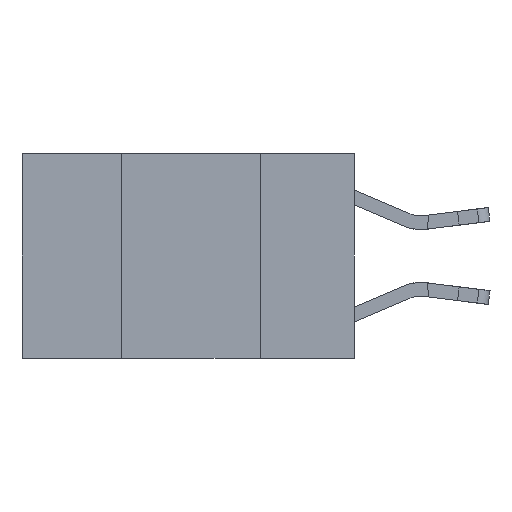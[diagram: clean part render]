
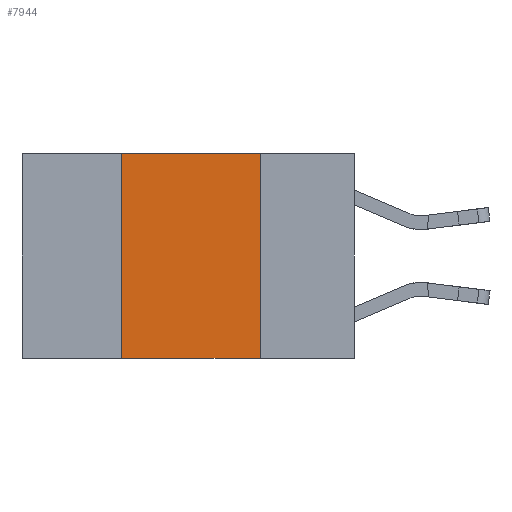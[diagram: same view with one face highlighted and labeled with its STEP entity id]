
A CAD part, left-side view. The second image highlights one B-rep face of the part: STEP entity #7944.
In plain terms, the highlighted planar face has unit normal (-1, 0, 0).
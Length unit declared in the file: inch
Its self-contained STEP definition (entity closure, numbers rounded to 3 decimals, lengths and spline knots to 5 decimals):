
#460 = AXIS2_PLACEMENT_3D ( 'NONE', #2028, #8259, #6343 ) ;
#480 = EDGE_LOOP ( 'NONE', ( #15426, #9861, #7995, #4561 ) ) ;
#1765 = CARTESIAN_POINT ( 'NONE',  ( 0., 0.42, -0.37 ) ) ;
#1944 = EDGE_CURVE ( 'NONE', #5459, #6682, #3910, .T. ) ;
#2028 = CARTESIAN_POINT ( 'NONE',  ( 0., 0.6, 0. ) ) ;
#2651 = CARTESIAN_POINT ( 'NONE',  ( 0., 0.42, 0. ) ) ;
#2825 = LINE ( 'NONE', #9179, #18843 ) ;
#3751 = DIRECTION ( 'NONE',  ( 0., 0., 1. ) ) ;
#3910 = LINE ( 'NONE', #19514, #7775 ) ;
#4037 = LINE ( 'NONE', #16080, #9561 ) ;
#4561 = ORIENTED_EDGE ( 'NONE', *, *, #10125, .T. ) ;
#5097 = FACE_OUTER_BOUND ( 'NONE', #480, .T. ) ;
#5459 = VERTEX_POINT ( 'NONE', #14041 ) ;
#6343 = DIRECTION ( 'NONE',  ( 0., 0., -1. ) ) ;
#6682 = VERTEX_POINT ( 'NONE', #13306 ) ;
#7086 = DIRECTION ( 'NONE',  ( 0., 0., -1. ) ) ;
#7775 = VECTOR ( 'NONE', #7086, 39.37008 ) ;
#7944 = ADVANCED_FACE ( 'NONE', ( #5097 ), #15928, .F. ) ;
#7995 = ORIENTED_EDGE ( 'NONE', *, *, #13094, .F. ) ;
#8259 = DIRECTION ( 'NONE',  ( 1., 0., 0. ) ) ;
#9179 = CARTESIAN_POINT ( 'NONE',  ( 0., 0.6, -0.37 ) ) ;
#9561 = VECTOR ( 'NONE', #19205, 39.37008 ) ;
#9861 = ORIENTED_EDGE ( 'NONE', *, *, #10482, .F. ) ;
#10125 = EDGE_CURVE ( 'NONE', #13511, #6682, #2825, .T. ) ;
#10482 = EDGE_CURVE ( 'NONE', #17206, #5459, #4037, .T. ) ;
#10518 = DIRECTION ( 'NONE',  ( 0., -1., 0. ) ) ;
#13094 = EDGE_CURVE ( 'NONE', #13511, #17206, #16112, .T. ) ;
#13306 = CARTESIAN_POINT ( 'NONE',  ( 0., 0.17, -0.37 ) ) ;
#13511 = VERTEX_POINT ( 'NONE', #1765 ) ;
#14041 = CARTESIAN_POINT ( 'NONE',  ( 0., 0.17, 0. ) ) ;
#15426 = ORIENTED_EDGE ( 'NONE', *, *, #1944, .F. ) ;
#15928 = PLANE ( 'NONE',  #460 ) ;
#16018 = VECTOR ( 'NONE', #3751, 39.37008 ) ;
#16080 = CARTESIAN_POINT ( 'NONE',  ( 0., 0.6, 0. ) ) ;
#16112 = LINE ( 'NONE', #18842, #16018 ) ;
#17206 = VERTEX_POINT ( 'NONE', #2651 ) ;
#18842 = CARTESIAN_POINT ( 'NONE',  ( 0., 0.42, 0. ) ) ;
#18843 = VECTOR ( 'NONE', #10518, 39.37008 ) ;
#19205 = DIRECTION ( 'NONE',  ( 0., -1., 0. ) ) ;
#19514 = CARTESIAN_POINT ( 'NONE',  ( 0., 0.17, 0. ) ) ;
